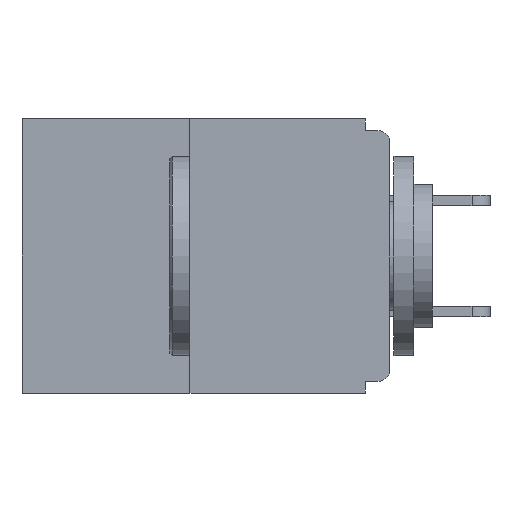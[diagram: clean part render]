
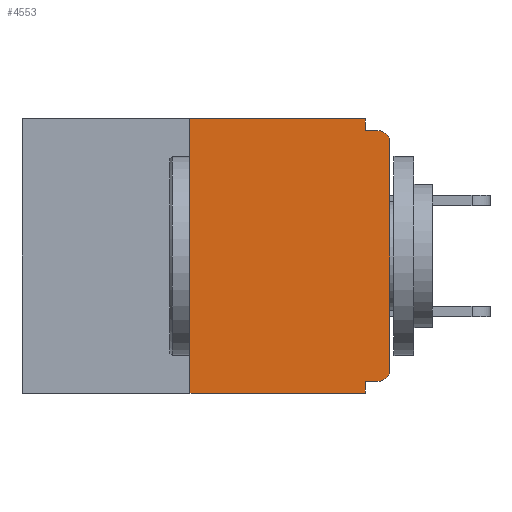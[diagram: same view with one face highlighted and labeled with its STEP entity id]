
A CAD part, left-side view. The second image highlights one B-rep face of the part: STEP entity #4553.
In plain terms, the highlighted planar face has unit normal (-1, 0, 0).
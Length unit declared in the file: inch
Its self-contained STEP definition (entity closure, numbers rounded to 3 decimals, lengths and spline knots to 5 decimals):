
#386 = DIRECTION ( 'NONE',  ( 0., 0., -1. ) ) ;
#983 = EDGE_LOOP ( 'NONE', ( #1333, #17315, #4181, #12941, #24377, #24673, #24652, #23739, #24287, #8205 ) ) ;
#1133 = DIRECTION ( 'NONE',  ( 1., 0., 0. ) ) ;
#1298 = CARTESIAN_POINT ( 'NONE',  ( 0., 0.031, 0. ) ) ;
#1318 = VERTEX_POINT ( 'NONE', #7290 ) ;
#1333 = ORIENTED_EDGE ( 'NONE', *, *, #14966, .F. ) ;
#1467 = VERTEX_POINT ( 'NONE', #5130 ) ;
#1532 = EDGE_CURVE ( 'NONE', #1318, #21279, #24384, .T. ) ;
#1614 = VECTOR ( 'NONE', #386, 39.37008 ) ;
#1943 = CARTESIAN_POINT ( 'NONE',  ( 0., 0., -0.328 ) ) ;
#2134 = DIRECTION ( 'NONE',  ( 0., 1., 0. ) ) ;
#2249 = VERTEX_POINT ( 'NONE', #26157 ) ;
#3179 = EDGE_CURVE ( 'NONE', #19457, #24314, #23175, .T. ) ;
#4181 = ORIENTED_EDGE ( 'NONE', *, *, #20693, .T. ) ;
#4553 = ADVANCED_FACE ( 'NONE', ( #15842 ), #21779, .F. ) ;
#4575 = LINE ( 'NONE', #6773, #15462 ) ;
#5130 = CARTESIAN_POINT ( 'NONE',  ( 0., 0.031, -0.328 ) ) ;
#5699 = CARTESIAN_POINT ( 'NONE',  ( 0., 0.031, 0. ) ) ;
#5773 = CARTESIAN_POINT ( 'NONE',  ( 0., 0.015, -0.015 ) ) ;
#5953 = DIRECTION ( 'NONE',  ( 0., 0., -1. ) ) ;
#6485 = VERTEX_POINT ( 'NONE', #5699 ) ;
#6578 = CARTESIAN_POINT ( 'NONE',  ( 0., 0.015, -0.03 ) ) ;
#6773 = CARTESIAN_POINT ( 'NONE',  ( 0., 0., -0.015 ) ) ;
#7092 = CARTESIAN_POINT ( 'NONE',  ( 0., 0.46, 0. ) ) ;
#7290 = CARTESIAN_POINT ( 'NONE',  ( 0., 0.015, -0.328 ) ) ;
#7802 = LINE ( 'NONE', #23573, #1614 ) ;
#8205 = ORIENTED_EDGE ( 'NONE', *, *, #9045, .F. ) ;
#9045 = EDGE_CURVE ( 'NONE', #6485, #15923, #13513, .T. ) ;
#9098 = LINE ( 'NONE', #27976, #19289 ) ;
#9120 = AXIS2_PLACEMENT_3D ( 'NONE', #12745, #15183, #22033 ) ;
#10529 = EDGE_CURVE ( 'NONE', #21279, #19457, #9098, .T. ) ;
#11139 = LINE ( 'NONE', #16329, #23110 ) ;
#12465 = VECTOR ( 'NONE', #13137, 39.37008 ) ;
#12632 = AXIS2_PLACEMENT_3D ( 'NONE', #6578, #20402, #15817 ) ;
#12745 = CARTESIAN_POINT ( 'NONE',  ( 0., 0.015, -0.313 ) ) ;
#12792 = VECTOR ( 'NONE', #5953, 39.37008 ) ;
#12941 = ORIENTED_EDGE ( 'NONE', *, *, #27602, .F. ) ;
#13137 = DIRECTION ( 'NONE',  ( 0., -1., 0. ) ) ;
#13513 = LINE ( 'NONE', #1298, #12792 ) ;
#13795 = LINE ( 'NONE', #29790, #21129 ) ;
#13969 = VERTEX_POINT ( 'NONE', #27177 ) ;
#14966 = EDGE_CURVE ( 'NONE', #2249, #6485, #20507, .T. ) ;
#15183 = DIRECTION ( 'NONE',  ( -1., 0., 0. ) ) ;
#15462 = VECTOR ( 'NONE', #24838, 39.37008 ) ;
#15817 = DIRECTION ( 'NONE',  ( 0., 0., -1. ) ) ;
#15842 = FACE_OUTER_BOUND ( 'NONE', #983, .T. ) ;
#15923 = VERTEX_POINT ( 'NONE', #18802 ) ;
#16083 = LINE ( 'NONE', #1943, #16418 ) ;
#16329 = CARTESIAN_POINT ( 'NONE',  ( 0., 0.46, -0.343 ) ) ;
#16418 = VECTOR ( 'NONE', #2134, 39.37008 ) ;
#17315 = ORIENTED_EDGE ( 'NONE', *, *, #17347, .F. ) ;
#17347 = EDGE_CURVE ( 'NONE', #13969, #2249, #13795, .T. ) ;
#17395 = DIRECTION ( 'NONE',  ( 0., 0., -1. ) ) ;
#18113 = CARTESIAN_POINT ( 'NONE',  ( 0., 0.031, -0.343 ) ) ;
#18253 = DIRECTION ( 'NONE',  ( 0., 0., 1. ) ) ;
#18802 = CARTESIAN_POINT ( 'NONE',  ( 0., 0.031, -0.015 ) ) ;
#19289 = VECTOR ( 'NONE', #23728, 39.37008 ) ;
#19457 = VERTEX_POINT ( 'NONE', #23770 ) ;
#20402 = DIRECTION ( 'NONE',  ( -1., 0., 0. ) ) ;
#20507 = LINE ( 'NONE', #7092, #12465 ) ;
#20656 = AXIS2_PLACEMENT_3D ( 'NONE', #24193, #1133, #17395 ) ;
#20693 = EDGE_CURVE ( 'NONE', #13969, #22204, #11139, .T. ) ;
#21045 = EDGE_CURVE ( 'NONE', #15923, #24314, #4575, .T. ) ;
#21129 = VECTOR ( 'NONE', #18253, 39.37008 ) ;
#21279 = VERTEX_POINT ( 'NONE', #25445 ) ;
#21779 = PLANE ( 'NONE',  #20656 ) ;
#22033 = DIRECTION ( 'NONE',  ( 0., 0., -1. ) ) ;
#22204 = VERTEX_POINT ( 'NONE', #18113 ) ;
#23110 = VECTOR ( 'NONE', #27803, 39.37008 ) ;
#23175 = CIRCLE ( 'NONE', #12632, 0.015 ) ;
#23392 = EDGE_CURVE ( 'NONE', #1318, #1467, #16083, .T. ) ;
#23573 = CARTESIAN_POINT ( 'NONE',  ( 0., 0.031, -0.343 ) ) ;
#23728 = DIRECTION ( 'NONE',  ( 0., 0., 1. ) ) ;
#23739 = ORIENTED_EDGE ( 'NONE', *, *, #3179, .T. ) ;
#23770 = CARTESIAN_POINT ( 'NONE',  ( 0., 0., -0.03 ) ) ;
#24193 = CARTESIAN_POINT ( 'NONE',  ( 0., 0.46, 0. ) ) ;
#24287 = ORIENTED_EDGE ( 'NONE', *, *, #21045, .F. ) ;
#24314 = VERTEX_POINT ( 'NONE', #5773 ) ;
#24377 = ORIENTED_EDGE ( 'NONE', *, *, #23392, .F. ) ;
#24384 = CIRCLE ( 'NONE', #9120, 0.015 ) ;
#24652 = ORIENTED_EDGE ( 'NONE', *, *, #10529, .T. ) ;
#24673 = ORIENTED_EDGE ( 'NONE', *, *, #1532, .T. ) ;
#24838 = DIRECTION ( 'NONE',  ( 0., -1., 0. ) ) ;
#25445 = CARTESIAN_POINT ( 'NONE',  ( 0., 0., -0.313 ) ) ;
#26157 = CARTESIAN_POINT ( 'NONE',  ( 0., 0.25, 0. ) ) ;
#27177 = CARTESIAN_POINT ( 'NONE',  ( 0., 0.25, -0.343 ) ) ;
#27602 = EDGE_CURVE ( 'NONE', #1467, #22204, #7802, .T. ) ;
#27803 = DIRECTION ( 'NONE',  ( 0., -1., 0. ) ) ;
#27976 = CARTESIAN_POINT ( 'NONE',  ( 0., 0., 0. ) ) ;
#29790 = CARTESIAN_POINT ( 'NONE',  ( 0., 0.25, 0. ) ) ;
